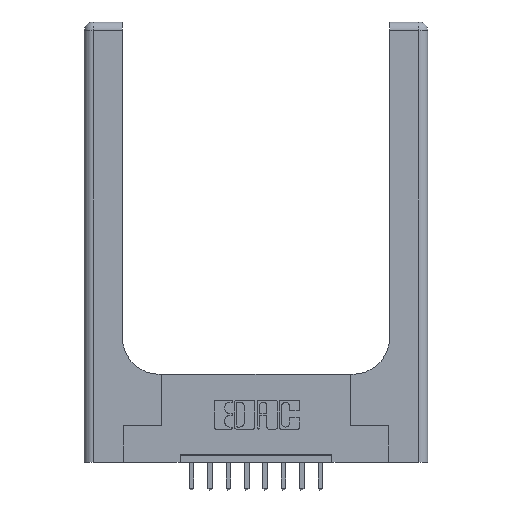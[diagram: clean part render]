
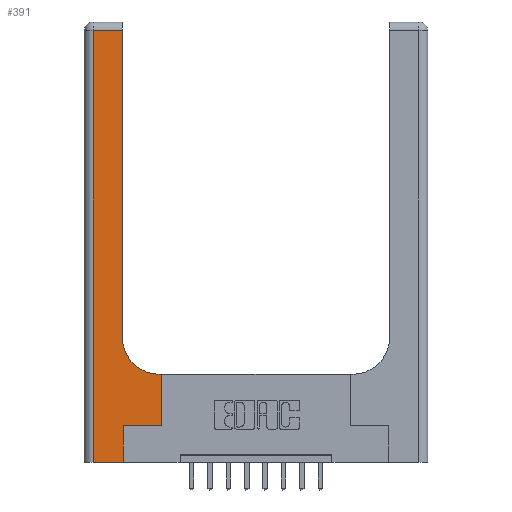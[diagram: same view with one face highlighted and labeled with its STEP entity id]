
A CAD part, top view. The second image highlights one B-rep face of the part: STEP entity #391.
In plain terms, the highlighted planar face has unit normal (0, 0, 1).
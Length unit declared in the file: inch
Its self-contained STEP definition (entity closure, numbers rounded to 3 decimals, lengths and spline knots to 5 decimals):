
#29 = ORIENTED_EDGE ( 'NONE', *, *, #5746, .T. ) ;
#163 = EDGE_CURVE ( 'NONE', #12926, #923, #4751, .T. ) ;
#297 = ORIENTED_EDGE ( 'NONE', *, *, #14818, .T. ) ;
#391 = ADVANCED_FACE ( 'NONE', ( #3660 ), #3234, .F. ) ;
#599 = DIRECTION ( 'NONE',  ( 0., -1., 0. ) ) ;
#672 = VECTOR ( 'NONE', #12549, 39.37008 ) ;
#673 = DIRECTION ( 'NONE',  ( 0., 0., -1. ) ) ;
#923 = VERTEX_POINT ( 'NONE', #5935 ) ;
#1205 = LINE ( 'NONE', #5316, #3346 ) ;
#1219 = CARTESIAN_POINT ( 'NONE',  ( 0.26, 0.6, 0.37 ) ) ;
#1580 = VERTEX_POINT ( 'NONE', #3577 ) ;
#1731 = EDGE_LOOP ( 'NONE', ( #10535, #297, #10408, #10460, #4535, #2621, #1864, #29, #7624 ) ) ;
#1806 = EDGE_CURVE ( 'NONE', #923, #5776, #7980, .T. ) ;
#1864 = ORIENTED_EDGE ( 'NONE', *, *, #13635, .T. ) ;
#2279 = LINE ( 'NONE', #5928, #672 ) ;
#2621 = ORIENTED_EDGE ( 'NONE', *, *, #9274, .T. ) ;
#2866 = VERTEX_POINT ( 'NONE', #3413 ) ;
#3049 = CIRCLE ( 'NONE', #8912, 0.25 ) ;
#3234 = PLANE ( 'NONE',  #3672 ) ;
#3346 = VECTOR ( 'NONE', #5418, 39.37008 ) ;
#3413 = CARTESIAN_POINT ( 'NONE',  ( 0.528, 0.25, 0.37 ) ) ;
#3530 = CARTESIAN_POINT ( 'NONE',  ( 0.26, 3., 0.37 ) ) ;
#3577 = CARTESIAN_POINT ( 'NONE',  ( 0.06, 2.94, 0.37 ) ) ;
#3660 = FACE_OUTER_BOUND ( 'NONE', #1731, .T. ) ;
#3672 = AXIS2_PLACEMENT_3D ( 'NONE', #7929, #673, #4008 ) ;
#3853 = CARTESIAN_POINT ( 'NONE',  ( 0.06, 0., 0.37 ) ) ;
#4008 = DIRECTION ( 'NONE',  ( -1., 0., 0. ) ) ;
#4535 = ORIENTED_EDGE ( 'NONE', *, *, #1806, .T. ) ;
#4628 = EDGE_CURVE ( 'NONE', #12388, #11213, #3049, .T. ) ;
#4751 = LINE ( 'NONE', #6927, #9064 ) ;
#5039 = CARTESIAN_POINT ( 'NONE',  ( 0.26, 0.85, 0.37 ) ) ;
#5115 = CARTESIAN_POINT ( 'NONE',  ( 0.51, 0.6, 0.37 ) ) ;
#5316 = CARTESIAN_POINT ( 'NONE',  ( 0., 2.94, 0.37 ) ) ;
#5418 = DIRECTION ( 'NONE',  ( -1., 0., 0. ) ) ;
#5742 = VECTOR ( 'NONE', #5989, 39.37008 ) ;
#5746 = EDGE_CURVE ( 'NONE', #13548, #12388, #7905, .T. ) ;
#5776 = VERTEX_POINT ( 'NONE', #10428 ) ;
#5928 = CARTESIAN_POINT ( 'NONE',  ( 0.265, 0.25, 0.37 ) ) ;
#5935 = CARTESIAN_POINT ( 'NONE',  ( 0.265, 0., 0.37 ) ) ;
#5989 = DIRECTION ( 'NONE',  ( -1., 0., 0. ) ) ;
#6009 = EDGE_CURVE ( 'NONE', #11213, #8947, #14836, .T. ) ;
#6397 = CARTESIAN_POINT ( 'NONE',  ( 0.06, 3., 0.37 ) ) ;
#6927 = CARTESIAN_POINT ( 'NONE',  ( 0., 0., 0.37 ) ) ;
#7384 = CARTESIAN_POINT ( 'NONE',  ( 0.265, 0., 0.37 ) ) ;
#7603 = DIRECTION ( 'NONE',  ( 1., 0., 0. ) ) ;
#7624 = ORIENTED_EDGE ( 'NONE', *, *, #4628, .T. ) ;
#7905 = LINE ( 'NONE', #1219, #5742 ) ;
#7929 = CARTESIAN_POINT ( 'NONE',  ( 0., 3., 0.37 ) ) ;
#7980 = LINE ( 'NONE', #7384, #12586 ) ;
#8486 = DIRECTION ( 'NONE',  ( 0., 1., 0. ) ) ;
#8792 = DIRECTION ( 'NONE',  ( 0., 0., -1. ) ) ;
#8912 = AXIS2_PLACEMENT_3D ( 'NONE', #12033, #8792, #7603 ) ;
#8947 = VERTEX_POINT ( 'NONE', #12060 ) ;
#9064 = VECTOR ( 'NONE', #11471, 39.37008 ) ;
#9274 = EDGE_CURVE ( 'NONE', #5776, #2866, #2279, .T. ) ;
#9320 = LINE ( 'NONE', #6397, #13082 ) ;
#9465 = VECTOR ( 'NONE', #11448, 39.37008 ) ;
#9747 = DIRECTION ( 'NONE',  ( 0., 1., 0. ) ) ;
#10408 = ORIENTED_EDGE ( 'NONE', *, *, #12524, .T. ) ;
#10428 = CARTESIAN_POINT ( 'NONE',  ( 0.265, 0.25, 0.37 ) ) ;
#10460 = ORIENTED_EDGE ( 'NONE', *, *, #163, .T. ) ;
#10535 = ORIENTED_EDGE ( 'NONE', *, *, #6009, .T. ) ;
#10800 = CARTESIAN_POINT ( 'NONE',  ( 0.528, 0.25, 0.37 ) ) ;
#11213 = VERTEX_POINT ( 'NONE', #5039 ) ;
#11448 = DIRECTION ( 'NONE',  ( 0., 1., 0. ) ) ;
#11471 = DIRECTION ( 'NONE',  ( 1., 0., 0. ) ) ;
#11987 = VECTOR ( 'NONE', #9747, 39.37008 ) ;
#12033 = CARTESIAN_POINT ( 'NONE',  ( 0.51, 0.85, 0.37 ) ) ;
#12060 = CARTESIAN_POINT ( 'NONE',  ( 0.26, 2.94, 0.37 ) ) ;
#12388 = VERTEX_POINT ( 'NONE', #5115 ) ;
#12524 = EDGE_CURVE ( 'NONE', #1580, #12926, #9320, .T. ) ;
#12549 = DIRECTION ( 'NONE',  ( 1., 0., 0. ) ) ;
#12586 = VECTOR ( 'NONE', #8486, 39.37008 ) ;
#12771 = CARTESIAN_POINT ( 'NONE',  ( 0.528, 0.6, 0.37 ) ) ;
#12857 = LINE ( 'NONE', #10800, #11987 ) ;
#12926 = VERTEX_POINT ( 'NONE', #3853 ) ;
#13082 = VECTOR ( 'NONE', #599, 39.37008 ) ;
#13548 = VERTEX_POINT ( 'NONE', #12771 ) ;
#13635 = EDGE_CURVE ( 'NONE', #2866, #13548, #12857, .T. ) ;
#14818 = EDGE_CURVE ( 'NONE', #8947, #1580, #1205, .T. ) ;
#14836 = LINE ( 'NONE', #3530, #9465 ) ;
